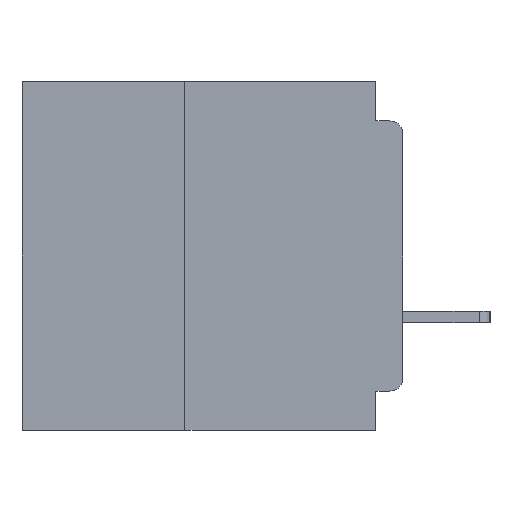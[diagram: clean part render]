
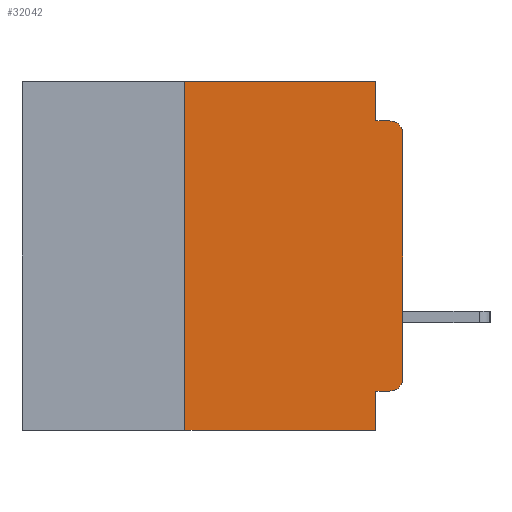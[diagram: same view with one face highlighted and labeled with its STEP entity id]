
A CAD part, left-side view. The second image highlights one B-rep face of the part: STEP entity #32042.
In plain terms, the highlighted planar face has unit normal (-1, 0, 0).
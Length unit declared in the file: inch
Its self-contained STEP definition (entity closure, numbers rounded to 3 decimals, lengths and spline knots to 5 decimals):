
#143 = LINE ( 'NONE', #6044, #8709 ) ;
#170 = CARTESIAN_POINT ( 'NONE',  ( 0., 0.015, -0.045 ) ) ;
#1001 = CARTESIAN_POINT ( 'NONE',  ( 0., 0.031, -0.355 ) ) ;
#1248 = CARTESIAN_POINT ( 'NONE',  ( 0., 0., -0.06 ) ) ;
#1250 = ORIENTED_EDGE ( 'NONE', *, *, #37970, .T. ) ;
#1386 = EDGE_CURVE ( 'NONE', #32647, #36421, #11420, .T. ) ;
#1670 = DIRECTION ( 'NONE',  ( -1., 0., 0. ) ) ;
#1712 = CARTESIAN_POINT ( 'NONE',  ( 0., 0.015, -0.355 ) ) ;
#1785 = EDGE_CURVE ( 'NONE', #8279, #42122, #13152, .T. ) ;
#2381 = DIRECTION ( 'NONE',  ( 0., 0., -1. ) ) ;
#2902 = PLANE ( 'NONE',  #32862 ) ;
#3160 = EDGE_CURVE ( 'NONE', #15063, #11341, #37053, .T. ) ;
#3733 = CARTESIAN_POINT ( 'NONE',  ( 0., 0., 0. ) ) ;
#5157 = EDGE_CURVE ( 'NONE', #36421, #26858, #35183, .T. ) ;
#5738 = LINE ( 'NONE', #26600, #13164 ) ;
#6044 = CARTESIAN_POINT ( 'NONE',  ( 0., 0.031, -0.4 ) ) ;
#7364 = DIRECTION ( 'NONE',  ( 0., 0., 1. ) ) ;
#8279 = VERTEX_POINT ( 'NONE', #24513 ) ;
#8433 = VECTOR ( 'NONE', #36740, 39.37008 ) ;
#8709 = VECTOR ( 'NONE', #2381, 39.37008 ) ;
#8765 = ORIENTED_EDGE ( 'NONE', *, *, #5157, .F. ) ;
#9314 = EDGE_CURVE ( 'NONE', #15063, #8279, #33838, .T. ) ;
#11341 = VERTEX_POINT ( 'NONE', #1001 ) ;
#11420 = LINE ( 'NONE', #40784, #28187 ) ;
#11451 = EDGE_LOOP ( 'NONE', ( #18274, #16858, #13793, #8765, #35831, #23994, #1250, #17430, #39843, #13862 ) ) ;
#12461 = CARTESIAN_POINT ( 'NONE',  ( 0., 0.031, -0.4 ) ) ;
#12700 = DIRECTION ( 'NONE',  ( -1., 0., 0. ) ) ;
#13152 = LINE ( 'NONE', #3733, #39421 ) ;
#13164 = VECTOR ( 'NONE', #37419, 39.37008 ) ;
#13793 = ORIENTED_EDGE ( 'NONE', *, *, #25944, .F. ) ;
#13862 = ORIENTED_EDGE ( 'NONE', *, *, #9314, .T. ) ;
#14658 = DIRECTION ( 'NONE',  ( 0., 0., -1. ) ) ;
#15063 = VERTEX_POINT ( 'NONE', #1712 ) ;
#16858 = ORIENTED_EDGE ( 'NONE', *, *, #24035, .T. ) ;
#17430 = ORIENTED_EDGE ( 'NONE', *, *, #21880, .F. ) ;
#18274 = ORIENTED_EDGE ( 'NONE', *, *, #1785, .T. ) ;
#19009 = CARTESIAN_POINT ( 'NONE',  ( 0., 0.031, -0.045 ) ) ;
#19830 = CARTESIAN_POINT ( 'NONE',  ( 0., 0.25, -0.4 ) ) ;
#20616 = CARTESIAN_POINT ( 'NONE',  ( 0., 0.031, 0. ) ) ;
#21016 = CARTESIAN_POINT ( 'NONE',  ( 0., 0.437, 0. ) ) ;
#21880 = EDGE_CURVE ( 'NONE', #11341, #45664, #143, .T. ) ;
#22389 = VERTEX_POINT ( 'NONE', #19830 ) ;
#22573 = CARTESIAN_POINT ( 'NONE',  ( 0., 0.25, -0.4 ) ) ;
#23347 = CARTESIAN_POINT ( 'NONE',  ( 0., 0.015, -0.34 ) ) ;
#23994 = ORIENTED_EDGE ( 'NONE', *, *, #25078, .F. ) ;
#24035 = EDGE_CURVE ( 'NONE', #42122, #41916, #44840, .T. ) ;
#24513 = CARTESIAN_POINT ( 'NONE',  ( 0., 0., -0.34 ) ) ;
#25078 = EDGE_CURVE ( 'NONE', #22389, #32647, #28119, .T. ) ;
#25944 = EDGE_CURVE ( 'NONE', #26858, #41916, #43603, .T. ) ;
#26600 = CARTESIAN_POINT ( 'NONE',  ( 0., 0.437, -0.4 ) ) ;
#26858 = VERTEX_POINT ( 'NONE', #19009 ) ;
#26894 = DIRECTION ( 'NONE',  ( 0., 0., -1. ) ) ;
#26985 = VECTOR ( 'NONE', #29698, 39.37008 ) ;
#28080 = DIRECTION ( 'NONE',  ( 0., 0., -1. ) ) ;
#28119 = LINE ( 'NONE', #22573, #26985 ) ;
#28187 = VECTOR ( 'NONE', #36824, 39.37008 ) ;
#28837 = CARTESIAN_POINT ( 'NONE',  ( 0., 0.031, 0. ) ) ;
#29698 = DIRECTION ( 'NONE',  ( 0., 0., 1. ) ) ;
#31369 = DIRECTION ( 'NONE',  ( 0., -1., 0. ) ) ;
#32042 = ADVANCED_FACE ( 'NONE', ( #42293 ), #2902, .F. ) ;
#32647 = VERTEX_POINT ( 'NONE', #35567 ) ;
#32862 = AXIS2_PLACEMENT_3D ( 'NONE', #21016, #38723, #28080 ) ;
#32922 = VECTOR ( 'NONE', #14658, 39.37008 ) ;
#33145 = CARTESIAN_POINT ( 'NONE',  ( 0., 0., -0.355 ) ) ;
#33838 = CIRCLE ( 'NONE', #44311, 0.015 ) ;
#34129 = CARTESIAN_POINT ( 'NONE',  ( 0., 0.015, -0.06 ) ) ;
#34200 = VECTOR ( 'NONE', #31369, 39.37008 ) ;
#35183 = LINE ( 'NONE', #28837, #32922 ) ;
#35567 = CARTESIAN_POINT ( 'NONE',  ( 0., 0.25, 0. ) ) ;
#35831 = ORIENTED_EDGE ( 'NONE', *, *, #1386, .F. ) ;
#36421 = VERTEX_POINT ( 'NONE', #20616 ) ;
#36740 = DIRECTION ( 'NONE',  ( 0., 1., 0. ) ) ;
#36824 = DIRECTION ( 'NONE',  ( 0., -1., 0. ) ) ;
#37053 = LINE ( 'NONE', #33145, #8433 ) ;
#37103 = AXIS2_PLACEMENT_3D ( 'NONE', #34129, #12700, #37721 ) ;
#37419 = DIRECTION ( 'NONE',  ( 0., -1., 0. ) ) ;
#37721 = DIRECTION ( 'NONE',  ( 0., 0., -1. ) ) ;
#37970 = EDGE_CURVE ( 'NONE', #22389, #45664, #5738, .T. ) ;
#38723 = DIRECTION ( 'NONE',  ( 1., 0., 0. ) ) ;
#39421 = VECTOR ( 'NONE', #7364, 39.37008 ) ;
#39843 = ORIENTED_EDGE ( 'NONE', *, *, #3160, .F. ) ;
#40784 = CARTESIAN_POINT ( 'NONE',  ( 0., 0.437, 0. ) ) ;
#41916 = VERTEX_POINT ( 'NONE', #170 ) ;
#42122 = VERTEX_POINT ( 'NONE', #1248 ) ;
#42293 = FACE_OUTER_BOUND ( 'NONE', #11451, .T. ) ;
#43603 = LINE ( 'NONE', #45642, #34200 ) ;
#44311 = AXIS2_PLACEMENT_3D ( 'NONE', #23347, #1670, #26894 ) ;
#44840 = CIRCLE ( 'NONE', #37103, 0.015 ) ;
#45642 = CARTESIAN_POINT ( 'NONE',  ( 0., 0., -0.045 ) ) ;
#45664 = VERTEX_POINT ( 'NONE', #12461 ) ;
